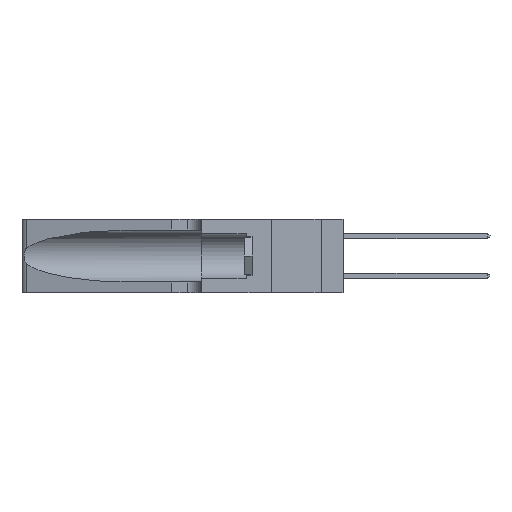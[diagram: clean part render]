
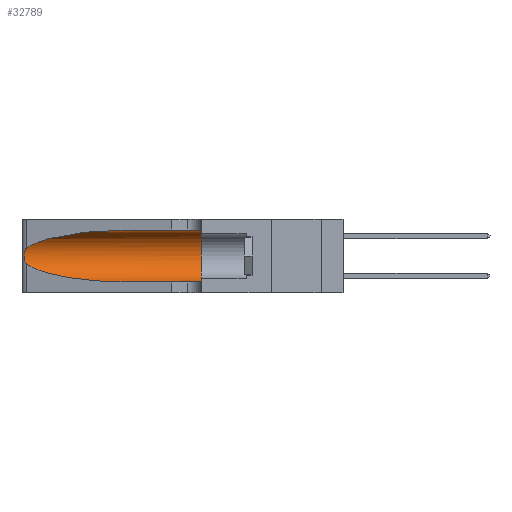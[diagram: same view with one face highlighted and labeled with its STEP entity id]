
A CAD part, left-side view. The second image highlights one B-rep face of the part: STEP entity #32789.
In plain terms, the highlighted cylindrical face has radius 3.308 mm (diameter 6.617 mm), a partial arc.
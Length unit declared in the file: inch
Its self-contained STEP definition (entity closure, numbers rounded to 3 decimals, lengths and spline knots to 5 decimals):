
#112 = CARTESIAN_POINT ( 'NONE',  ( 0.26017, 1.23833, 0.17102 ) ) ;
#208 = CARTESIAN_POINT ( 'NONE',  ( 0.25854, 1.2359, 0.20912 ) ) ;
#239 = AXIS2_PLACEMENT_3D ( 'NONE', #32086, #26904, #24470 ) ;
#728 = CARTESIAN_POINT ( 'NONE',  ( 0.1305, 0.72297, 0.05475 ) ) ;
#1362 = CARTESIAN_POINT ( 'NONE',  ( 0.1305, 0.35, 0.185 ) ) ;
#2537 = EDGE_CURVE ( 'NONE', #7131, #3414, #5963, .T. ) ;
#2668 = CARTESIAN_POINT ( 'NONE',  ( 0.25789, 1.23486, 0.15765 ) ) ;
#2888 = CARTESIAN_POINT ( 'NONE',  ( 0.25555, 1.22993, 0.14849 ) ) ;
#2890 = DIRECTION ( 'NONE',  ( 0., -1., 0. ) ) ;
#3164 = CARTESIAN_POINT ( 'NONE',  ( 0.25487, 1.22718, 0.22369 ) ) ;
#3183 = EDGE_CURVE ( 'NONE', #11620, #7131, #31779, .T. ) ;
#3352 = ORIENTED_EDGE ( 'NONE', *, *, #2537, .T. ) ;
#3414 = VERTEX_POINT ( 'NONE', #9869 ) ;
#4843 = CIRCLE ( 'NONE', #28712, 0.13025 ) ;
#4921 = VERTEX_POINT ( 'NONE', #7850 ) ;
#4936 = CARTESIAN_POINT ( 'NONE',  ( 0.2373, 1.15595, 0.08982 ) ) ;
#5262 = CARTESIAN_POINT ( 'NONE',  ( 0.25555, 1.22994, 0.2215 ) ) ;
#5359 = CARTESIAN_POINT ( 'NONE',  ( 0.25487, 1.22718, 0.14631 ) ) ;
#5963 = B_SPLINE_CURVE_WITH_KNOTS ( 'NONE', 3,
 ( #20899, #5262, #25814, #18249, #208, #25711, #20689, #13111, #112, #23374, #2668, #10551, #2888, #5359 ),
 .UNSPECIFIED., .F., .F.,
 ( 4, 2, 2, 2, 2, 2, 4 ),
 ( 0., 0.00027, 0.00053, 0.00107, 0.0016, 0.00187, 0.00214 ),
 .UNSPECIFIED. ) ;
#6295 = LINE ( 'NONE', #30786, #27539 ) ;
#6547 = VECTOR ( 'NONE', #2890, 39.37008 ) ;
#6630 =( BOUNDED_CURVE ( )  B_SPLINE_CURVE ( 3, ( #30179, #4936, #27383, #7055 ),
 .UNSPECIFIED., .F., .F. ) 
 B_SPLINE_CURVE_WITH_KNOTS ( ( 4, 4 ),
 ( 3.44316, 4.71239 ),
 .UNSPECIFIED. ) 
 CURVE ( )  GEOMETRIC_REPRESENTATION_ITEM ( )  RATIONAL_B_SPLINE_CURVE ( ( 1., 0.87, 0.87, 1. ) ) 
 REPRESENTATION_ITEM ( '' )  );
#6776 = EDGE_CURVE ( 'NONE', #3414, #17088, #6630, .T. ) ;
#7055 = CARTESIAN_POINT ( 'NONE',  ( 0.1305, 0.72297, 0.05475 ) ) ;
#7131 = VERTEX_POINT ( 'NONE', #15645 ) ;
#7680 = DIRECTION ( 'NONE',  ( 0., -1., 0. ) ) ;
#7850 = CARTESIAN_POINT ( 'NONE',  ( 0.1305, 0.35, 0.31525 ) ) ;
#8030 = CARTESIAN_POINT ( 'NONE',  ( 0.1305, 0.72297, 0.31525 ) ) ;
#8658 = DIRECTION ( 'NONE',  ( 0., 1., 0. ) ) ;
#9160 = EDGE_CURVE ( 'NONE', #4921, #14750, #4843, .T. ) ;
#9869 = CARTESIAN_POINT ( 'NONE',  ( 0.25487, 1.22718, 0.14631 ) ) ;
#10439 = EDGE_CURVE ( 'NONE', #11620, #4921, #6295, .T. ) ;
#10551 = CARTESIAN_POINT ( 'NONE',  ( 0.25639, 1.23186, 0.15144 ) ) ;
#11620 = VERTEX_POINT ( 'NONE', #28087 ) ;
#12242 = LINE ( 'NONE', #28178, #6547 ) ;
#13111 = CARTESIAN_POINT ( 'NONE',  ( 0.26075, 1.23896, 0.178 ) ) ;
#14750 = VERTEX_POINT ( 'NONE', #28993 ) ;
#15645 = CARTESIAN_POINT ( 'NONE',  ( 0.25487, 1.22718, 0.22369 ) ) ;
#15920 = ORIENTED_EDGE ( 'NONE', *, *, #10439, .F. ) ;
#17088 = VERTEX_POINT ( 'NONE', #728 ) ;
#17799 = ORIENTED_EDGE ( 'NONE', *, *, #30583, .T. ) ;
#18249 = CARTESIAN_POINT ( 'NONE',  ( 0.25787, 1.23484, 0.2124 ) ) ;
#19073 = DIRECTION ( 'NONE',  ( 0., 0., 1. ) ) ;
#20689 = CARTESIAN_POINT ( 'NONE',  ( 0.26075, 1.23896, 0.19203 ) ) ;
#20861 = CARTESIAN_POINT ( 'NONE',  ( 0.18966, 0.96281, 0.31525 ) ) ;
#20899 = CARTESIAN_POINT ( 'NONE',  ( 0.25487, 1.22718, 0.22369 ) ) ;
#21025 = ORIENTED_EDGE ( 'NONE', *, *, #6776, .T. ) ;
#21076 = CARTESIAN_POINT ( 'NONE',  ( 0.2373, 1.15595, 0.28018 ) ) ;
#22908 = ORIENTED_EDGE ( 'NONE', *, *, #9160, .F. ) ;
#23374 = CARTESIAN_POINT ( 'NONE',  ( 0.25856, 1.23593, 0.16098 ) ) ;
#24470 = DIRECTION ( 'NONE',  ( 0., 0., -1. ) ) ;
#25576 = ORIENTED_EDGE ( 'NONE', *, *, #3183, .T. ) ;
#25711 = CARTESIAN_POINT ( 'NONE',  ( 0.26018, 1.23835, 0.19895 ) ) ;
#25814 = CARTESIAN_POINT ( 'NONE',  ( 0.25639, 1.23184, 0.21858 ) ) ;
#26523 = CYLINDRICAL_SURFACE ( 'NONE', #239, 0.13025 ) ;
#26904 = DIRECTION ( 'NONE',  ( 0., -1., 0. ) ) ;
#27383 = CARTESIAN_POINT ( 'NONE',  ( 0.18966, 0.96281, 0.05475 ) ) ;
#27439 = EDGE_LOOP ( 'NONE', ( #25576, #3352, #21025, #17799, #22908, #15920 ) ) ;
#27539 = VECTOR ( 'NONE', #7680, 39.37008 ) ;
#28087 = CARTESIAN_POINT ( 'NONE',  ( 0.1305, 0.72297, 0.31525 ) ) ;
#28178 = CARTESIAN_POINT ( 'NONE',  ( 0.1305, 1.61858, 0.05475 ) ) ;
#28712 = AXIS2_PLACEMENT_3D ( 'NONE', #1362, #8658, #19073 ) ;
#28993 = CARTESIAN_POINT ( 'NONE',  ( 0.1305, 0.35, 0.05475 ) ) ;
#30179 = CARTESIAN_POINT ( 'NONE',  ( 0.25487, 1.22718, 0.14631 ) ) ;
#30578 = FACE_OUTER_BOUND ( 'NONE', #27439, .T. ) ;
#30583 = EDGE_CURVE ( 'NONE', #17088, #14750, #12242, .T. ) ;
#30786 = CARTESIAN_POINT ( 'NONE',  ( 0.1305, 1.61858, 0.31525 ) ) ;
#31779 =( BOUNDED_CURVE ( )  B_SPLINE_CURVE ( 3, ( #8030, #20861, #21076, #3164 ),
 .UNSPECIFIED., .F., .T. ) 
 B_SPLINE_CURVE_WITH_KNOTS ( ( 4, 4 ),
 ( 1.5708, 2.84003 ),
 .UNSPECIFIED. ) 
 CURVE ( )  GEOMETRIC_REPRESENTATION_ITEM ( )  RATIONAL_B_SPLINE_CURVE ( ( 1., 0.87, 0.87, 1. ) ) 
 REPRESENTATION_ITEM ( '' )  );
#32086 = CARTESIAN_POINT ( 'NONE',  ( 0.1305, 1.61858, 0.185 ) ) ;
#32789 = ADVANCED_FACE ( 'NONE', ( #30578 ), #26523, .F. ) ;
